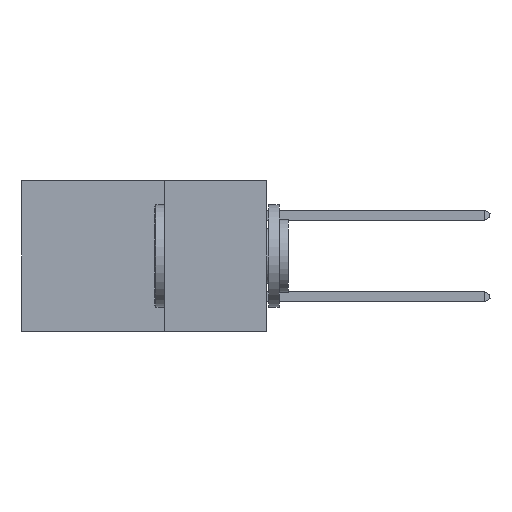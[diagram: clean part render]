
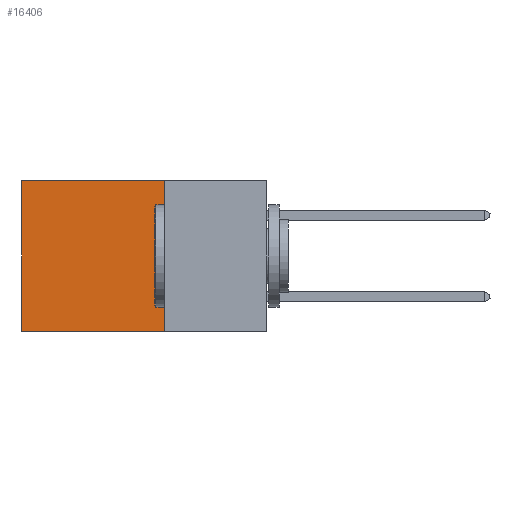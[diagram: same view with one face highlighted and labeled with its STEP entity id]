
A CAD part, left-side view. The second image highlights one B-rep face of the part: STEP entity #16406.
In plain terms, the highlighted planar face has unit normal (-1, 0, 0).
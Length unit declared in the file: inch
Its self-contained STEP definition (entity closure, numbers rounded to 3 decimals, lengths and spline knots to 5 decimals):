
#681 = CARTESIAN_POINT ( 'NONE',  ( 0.2875, 0.25, 0. ) ) ;
#1119 = LINE ( 'NONE', #31741, #17788 ) ;
#3461 = ORIENTED_EDGE ( 'NONE', *, *, #20181, .T. ) ;
#4446 = CARTESIAN_POINT ( 'NONE',  ( 0.2875, 0.25, 0. ) ) ;
#5886 = DIRECTION ( 'NONE',  ( 0., 1., 0. ) ) ;
#8870 = EDGE_CURVE ( 'NONE', #32077, #16356, #19377, .T. ) ;
#9573 = EDGE_CURVE ( 'NONE', #33086, #16284, #31115, .T. ) ;
#9996 = VECTOR ( 'NONE', #30030, 39.37008 ) ;
#12397 = PLANE ( 'NONE',  #26488 ) ;
#16284 = VERTEX_POINT ( 'NONE', #24730 ) ;
#16356 = VERTEX_POINT ( 'NONE', #24920 ) ;
#16406 = ADVANCED_FACE ( 'NONE', ( #30206 ), #12397, .F. ) ;
#16577 = ORIENTED_EDGE ( 'NONE', *, *, #17675, .F. ) ;
#17155 = CARTESIAN_POINT ( 'NONE',  ( 0.2875, 0.25, 0. ) ) ;
#17179 = DIRECTION ( 'NONE',  ( 0., 0., -1. ) ) ;
#17416 = DIRECTION ( 'NONE',  ( 1., 0., 0. ) ) ;
#17675 = EDGE_CURVE ( 'NONE', #32077, #33086, #28901, .T. ) ;
#17788 = VECTOR ( 'NONE', #24148, 39.37008 ) ;
#18721 = VECTOR ( 'NONE', #19229, 39.37008 ) ;
#19229 = DIRECTION ( 'NONE',  ( 0., 0., -1. ) ) ;
#19377 = LINE ( 'NONE', #17155, #21020 ) ;
#20181 = EDGE_CURVE ( 'NONE', #16356, #16284, #1119, .T. ) ;
#21020 = VECTOR ( 'NONE', #5886, 39.37008 ) ;
#22632 = CARTESIAN_POINT ( 'NONE',  ( 0.2875, 0.25, 0. ) ) ;
#24148 = DIRECTION ( 'NONE',  ( 0., 0., -1. ) ) ;
#24192 = ORIENTED_EDGE ( 'NONE', *, *, #9573, .F. ) ;
#24271 = ORIENTED_EDGE ( 'NONE', *, *, #8870, .T. ) ;
#24730 = CARTESIAN_POINT ( 'NONE',  ( 0.2875, 0.6, -0.37 ) ) ;
#24920 = CARTESIAN_POINT ( 'NONE',  ( 0.2875, 0.6, 0. ) ) ;
#26110 = CARTESIAN_POINT ( 'NONE',  ( 0.2875, 0.25, -0.37 ) ) ;
#26488 = AXIS2_PLACEMENT_3D ( 'NONE', #4446, #17416, #17179 ) ;
#27305 = CARTESIAN_POINT ( 'NONE',  ( 0.2875, 0.25, -0.37 ) ) ;
#28776 = EDGE_LOOP ( 'NONE', ( #3461, #24192, #16577, #24271 ) ) ;
#28901 = LINE ( 'NONE', #681, #18721 ) ;
#30030 = DIRECTION ( 'NONE',  ( 0., 1., 0. ) ) ;
#30206 = FACE_OUTER_BOUND ( 'NONE', #28776, .T. ) ;
#31115 = LINE ( 'NONE', #27305, #9996 ) ;
#31741 = CARTESIAN_POINT ( 'NONE',  ( 0.2875, 0.6, 0. ) ) ;
#32077 = VERTEX_POINT ( 'NONE', #22632 ) ;
#33086 = VERTEX_POINT ( 'NONE', #26110 ) ;
